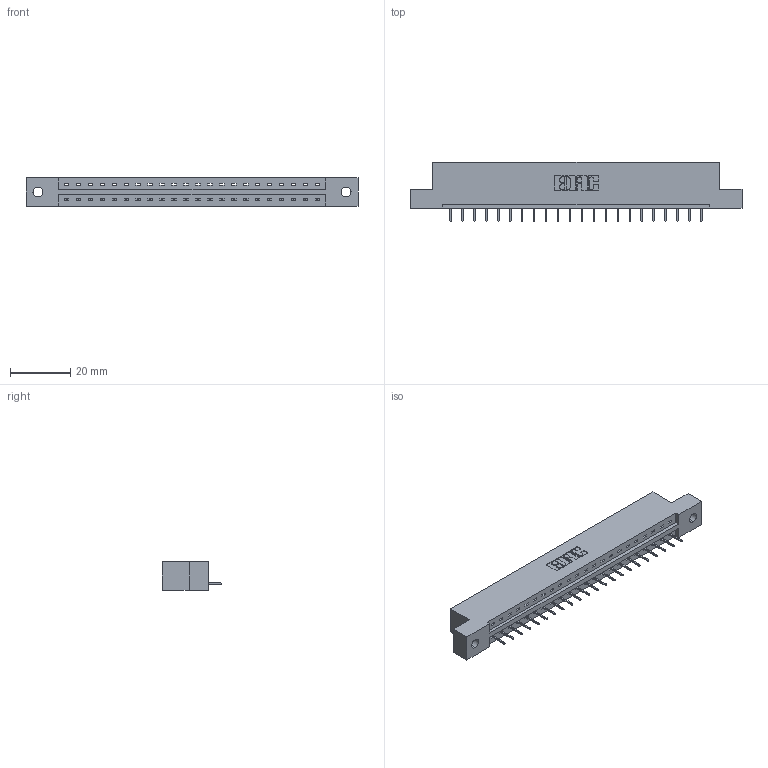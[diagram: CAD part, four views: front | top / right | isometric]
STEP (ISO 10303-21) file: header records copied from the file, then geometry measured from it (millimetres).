
FILE_DESCRIPTION (( 'STEP AP203' ), '1' );
FILE_NAME ('387-022-524-102.STEP', '2019-10-03T01:09:10', ( '' ), ( '' ), 'SwSTEP 2.0', 'SolidWorks 2016', '' );
FILE_SCHEMA (( 'CONFIG_CONTROL_DESIGN' ));
Length unit declared in the file: inch
Products named in the file (3): 345-292-001_345-293-124; 387-022-524-102; 337 Part_Flush Mounting Lugs - 0.128 Dia
Assembly tree (23 placements, depth 2):
  387-022-524-102
    337 Part_Flush Mounting Lugs - 0.128 Dia
    345-292-001_345-293-124  x22
Bounding box: 110.19 x 19.69 x 9.4 mm (x, y, z)
Volume: 11078 mm3; surface area: 10761 mm2
Topology: 23 solids, 23 shells, 1566 faces, 4535 edges, 2934 vertices
Faces by surface type: plane 1214, cylinder 352
Entity records: 19017 total; most frequent: CARTESIAN_POINT 3316, ORIENTED_EDGE 3274, DIRECTION 2833, EDGE_CURVE 1637, VECTOR 1513, LINE 1513, VERTEX_POINT 1086, AXIS2_PLACEMENT_3D 660
